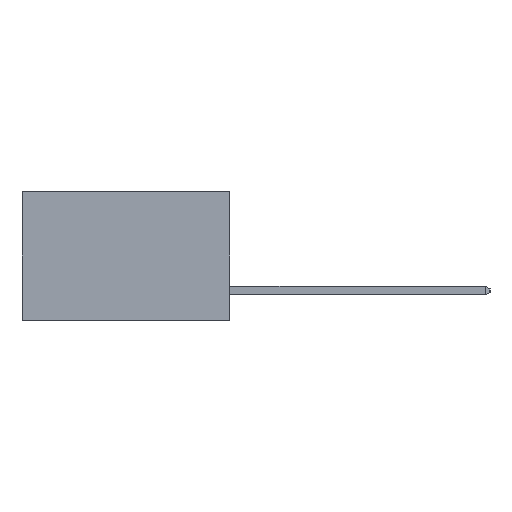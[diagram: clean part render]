
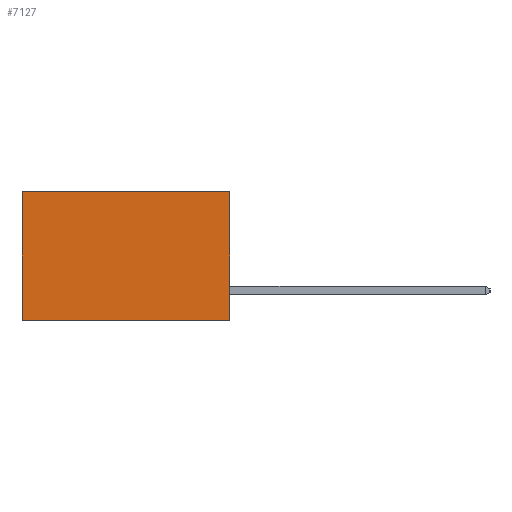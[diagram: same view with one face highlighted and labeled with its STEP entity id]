
A CAD part, left-side view. The second image highlights one B-rep face of the part: STEP entity #7127.
In plain terms, the highlighted planar face has unit normal (-1, 0, 0).
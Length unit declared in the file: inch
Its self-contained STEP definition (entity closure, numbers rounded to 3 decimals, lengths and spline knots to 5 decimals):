
#506 = VERTEX_POINT ( 'NONE', #9619 ) ;
#640 = DIRECTION ( 'NONE',  ( 0., 0., -1. ) ) ;
#847 = ORIENTED_EDGE ( 'NONE', *, *, #4577, .T. ) ;
#900 = CARTESIAN_POINT ( 'NONE',  ( 0.298, 0., -0.37 ) ) ;
#1030 = VECTOR ( 'NONE', #1803, 39.37008 ) ;
#1155 = CARTESIAN_POINT ( 'NONE',  ( 0.298, 0., 0. ) ) ;
#1327 = AXIS2_PLACEMENT_3D ( 'NONE', #10040, #8628, #8538 ) ;
#1358 = CARTESIAN_POINT ( 'NONE',  ( 0.298, 0., 0. ) ) ;
#1731 = VECTOR ( 'NONE', #6493, 39.37008 ) ;
#1803 = DIRECTION ( 'NONE',  ( 0., 1., 0. ) ) ;
#3047 = EDGE_LOOP ( 'NONE', ( #3736, #9531, #5642, #847 ) ) ;
#3131 = CARTESIAN_POINT ( 'NONE',  ( 0.298, 0., 0. ) ) ;
#3736 = ORIENTED_EDGE ( 'NONE', *, *, #10011, .T. ) ;
#3989 = EDGE_CURVE ( 'NONE', #6353, #4723, #7016, .T. ) ;
#4577 = EDGE_CURVE ( 'NONE', #6353, #8065, #9551, .T. ) ;
#4672 = VECTOR ( 'NONE', #640, 39.37008 ) ;
#4723 = VERTEX_POINT ( 'NONE', #6649 ) ;
#5426 = VECTOR ( 'NONE', #8501, 39.37008 ) ;
#5607 = FACE_OUTER_BOUND ( 'NONE', #3047, .T. ) ;
#5642 = ORIENTED_EDGE ( 'NONE', *, *, #3989, .F. ) ;
#5704 = CARTESIAN_POINT ( 'NONE',  ( 0.298, 0.6, 0. ) ) ;
#6353 = VERTEX_POINT ( 'NONE', #3131 ) ;
#6493 = DIRECTION ( 'NONE',  ( 0., 0., -1. ) ) ;
#6649 = CARTESIAN_POINT ( 'NONE',  ( 0.298, 0., -0.37 ) ) ;
#6948 = CARTESIAN_POINT ( 'NONE',  ( 0.298, 0.6, 0. ) ) ;
#7016 = LINE ( 'NONE', #1358, #4672 ) ;
#7127 = ADVANCED_FACE ( 'NONE', ( #5607 ), #9388, .F. ) ;
#7658 = LINE ( 'NONE', #900, #1030 ) ;
#8065 = VERTEX_POINT ( 'NONE', #6948 ) ;
#8271 = LINE ( 'NONE', #5704, #1731 ) ;
#8501 = DIRECTION ( 'NONE',  ( 0., 1., 0. ) ) ;
#8538 = DIRECTION ( 'NONE',  ( 0., 0., -1. ) ) ;
#8628 = DIRECTION ( 'NONE',  ( 1., 0., 0. ) ) ;
#9388 = PLANE ( 'NONE',  #1327 ) ;
#9531 = ORIENTED_EDGE ( 'NONE', *, *, #10246, .F. ) ;
#9551 = LINE ( 'NONE', #1155, #5426 ) ;
#9619 = CARTESIAN_POINT ( 'NONE',  ( 0.298, 0.6, -0.37 ) ) ;
#10011 = EDGE_CURVE ( 'NONE', #8065, #506, #8271, .T. ) ;
#10040 = CARTESIAN_POINT ( 'NONE',  ( 0.298, 0., 0. ) ) ;
#10246 = EDGE_CURVE ( 'NONE', #4723, #506, #7658, .T. ) ;
